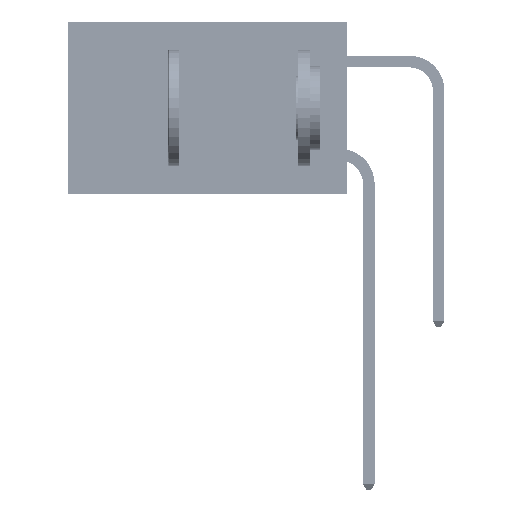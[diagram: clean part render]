
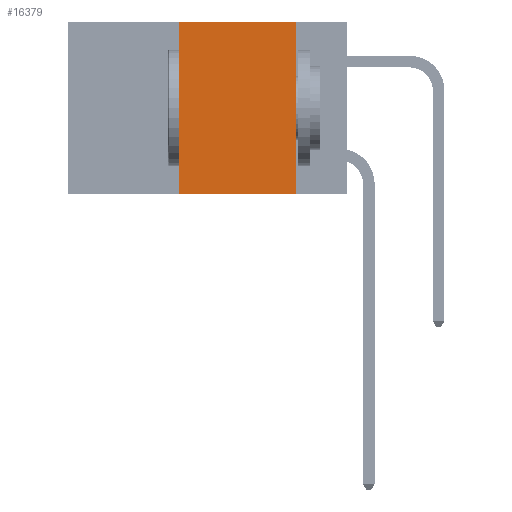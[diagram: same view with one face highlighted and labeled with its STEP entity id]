
A CAD part, left-side view. The second image highlights one B-rep face of the part: STEP entity #16379.
In plain terms, the highlighted planar face has unit normal (-1, 0, 0).
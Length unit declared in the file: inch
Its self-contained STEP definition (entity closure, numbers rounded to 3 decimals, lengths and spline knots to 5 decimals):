
#76 = EDGE_CURVE ( 'NONE', #31299, #10656, #6066, .T. ) ;
#1594 = PLANE ( 'NONE',  #32832 ) ;
#6066 = LINE ( 'NONE', #26608, #23938 ) ;
#9852 = DIRECTION ( 'NONE',  ( 1., 0., 0. ) ) ;
#10656 = VERTEX_POINT ( 'NONE', #31901 ) ;
#12178 = VERTEX_POINT ( 'NONE', #50337 ) ;
#12850 = CARTESIAN_POINT ( 'NONE',  ( 0., 0.11, 0. ) ) ;
#13857 = LINE ( 'NONE', #37180, #48452 ) ;
#16379 = ADVANCED_FACE ( 'NONE', ( #35807 ), #1594, .F. ) ;
#18257 = DIRECTION ( 'NONE',  ( 0., 0., -1. ) ) ;
#20642 = EDGE_CURVE ( 'NONE', #27704, #31299, #45004, .T. ) ;
#22907 = ORIENTED_EDGE ( 'NONE', *, *, #38095, .F. ) ;
#23938 = VECTOR ( 'NONE', #43066, 39.37008 ) ;
#24838 = ORIENTED_EDGE ( 'NONE', *, *, #76, .F. ) ;
#26608 = CARTESIAN_POINT ( 'NONE',  ( 0., 0.6, 0. ) ) ;
#27704 = VERTEX_POINT ( 'NONE', #38941 ) ;
#28602 = ORIENTED_EDGE ( 'NONE', *, *, #20642, .F. ) ;
#31299 = VERTEX_POINT ( 'NONE', #40050 ) ;
#31901 = CARTESIAN_POINT ( 'NONE',  ( 0., 0.11, 0. ) ) ;
#32832 = AXIS2_PLACEMENT_3D ( 'NONE', #34873, #9852, #18257 ) ;
#33945 = LINE ( 'NONE', #12850, #35893 ) ;
#34873 = CARTESIAN_POINT ( 'NONE',  ( 0., 0.6, 0. ) ) ;
#35223 = EDGE_LOOP ( 'NONE', ( #22907, #24838, #28602, #45134 ) ) ;
#35807 = FACE_OUTER_BOUND ( 'NONE', #35223, .T. ) ;
#35893 = VECTOR ( 'NONE', #41267, 39.37008 ) ;
#37180 = CARTESIAN_POINT ( 'NONE',  ( 0., 0.6, -0.37 ) ) ;
#37709 = DIRECTION ( 'NONE',  ( 0., 0., 1. ) ) ;
#38095 = EDGE_CURVE ( 'NONE', #10656, #12178, #33945, .T. ) ;
#38941 = CARTESIAN_POINT ( 'NONE',  ( 0., 0.36, -0.37 ) ) ;
#40050 = CARTESIAN_POINT ( 'NONE',  ( 0., 0.36, 0. ) ) ;
#41264 = DIRECTION ( 'NONE',  ( 0., -1., 0. ) ) ;
#41267 = DIRECTION ( 'NONE',  ( 0., 0., -1. ) ) ;
#43066 = DIRECTION ( 'NONE',  ( 0., -1., 0. ) ) ;
#45004 = LINE ( 'NONE', #52688, #49477 ) ;
#45134 = ORIENTED_EDGE ( 'NONE', *, *, #51494, .T. ) ;
#48452 = VECTOR ( 'NONE', #41264, 39.37008 ) ;
#49477 = VECTOR ( 'NONE', #37709, 39.37008 ) ;
#50337 = CARTESIAN_POINT ( 'NONE',  ( 0., 0.11, -0.37 ) ) ;
#51494 = EDGE_CURVE ( 'NONE', #27704, #12178, #13857, .T. ) ;
#52688 = CARTESIAN_POINT ( 'NONE',  ( 0., 0.36, 0. ) ) ;
